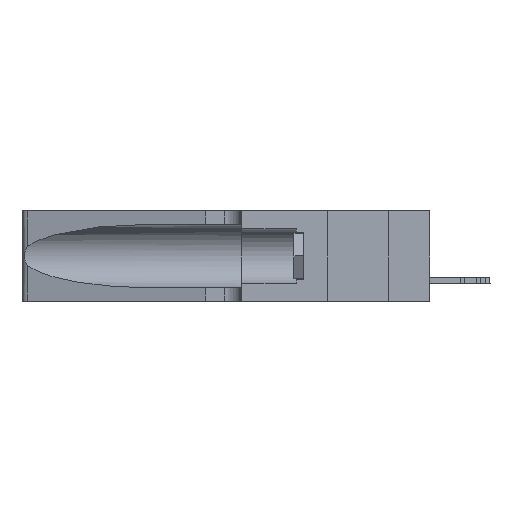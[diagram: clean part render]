
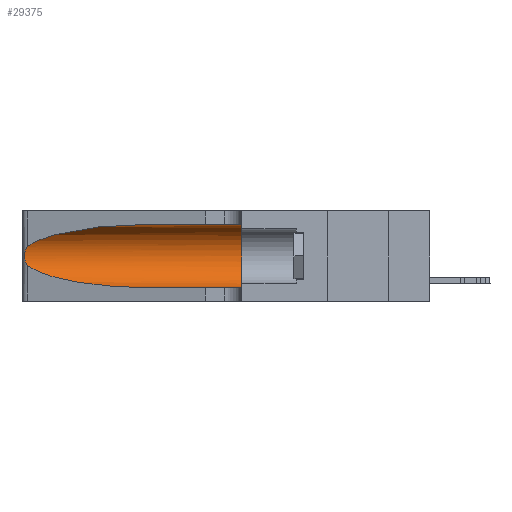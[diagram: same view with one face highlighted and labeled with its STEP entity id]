
A CAD part, left-side view. The second image highlights one B-rep face of the part: STEP entity #29375.
In plain terms, the highlighted cylindrical face has radius 3.308 mm (diameter 6.617 mm), a partial arc.
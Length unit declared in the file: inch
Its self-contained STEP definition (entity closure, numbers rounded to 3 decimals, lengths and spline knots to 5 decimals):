
#72 = CIRCLE ( 'NONE', #25936, 0.13025 ) ;
#590 =( BOUNDED_CURVE ( )  B_SPLINE_CURVE ( 3, ( #35340, #2138, #42446, #32160 ),
 .UNSPECIFIED., .F., .T. ) 
 B_SPLINE_CURVE_WITH_KNOTS ( ( 4, 4 ),
 ( 1.5708, 2.84003 ),
 .UNSPECIFIED. ) 
 CURVE ( )  GEOMETRIC_REPRESENTATION_ITEM ( )  RATIONAL_B_SPLINE_CURVE ( ( 1., 0.87, 0.87, 1. ) ) 
 REPRESENTATION_ITEM ( '' )  );
#1772 = CYLINDRICAL_SURFACE ( 'NONE', #24110, 0.13025 ) ;
#2138 = CARTESIAN_POINT ( 'NONE',  ( 0.18966, 0.96281, 0.31525 ) ) ;
#3364 = CARTESIAN_POINT ( 'NONE',  ( 0.26017, 1.23833, 0.17102 ) ) ;
#3553 = CARTESIAN_POINT ( 'NONE',  ( 0.1305, 0.72297, 0.05475 ) ) ;
#4095 = VERTEX_POINT ( 'NONE', #39929 ) ;
#5982 = CARTESIAN_POINT ( 'NONE',  ( 0.25639, 1.23184, 0.21858 ) ) ;
#6712 = CARTESIAN_POINT ( 'NONE',  ( 0.25787, 1.23484, 0.2124 ) ) ;
#8553 = B_SPLINE_CURVE_WITH_KNOTS ( 'NONE', 3,
 ( #29256, #28827, #5982, #6712, #12240, #23269, #42058, #12664, #3364, #29982, #9185, #25629, #38862, #39005 ),
 .UNSPECIFIED., .F., .F.,
 ( 4, 2, 2, 2, 2, 2, 4 ),
 ( 0., 0.00027, 0.00053, 0.00107, 0.0016, 0.00187, 0.00214 ),
 .UNSPECIFIED. ) ;
#9185 = CARTESIAN_POINT ( 'NONE',  ( 0.25789, 1.23486, 0.15765 ) ) ;
#10046 = CARTESIAN_POINT ( 'NONE',  ( 0.1305, 0.35, 0.05475 ) ) ;
#10356 = EDGE_CURVE ( 'NONE', #38696, #4095, #590, .T. ) ;
#10745 = CARTESIAN_POINT ( 'NONE',  ( 0.1305, 1.61858, 0.31525 ) ) ;
#10902 = CARTESIAN_POINT ( 'NONE',  ( 0.1305, 0.72297, 0.05475 ) ) ;
#11065 = VERTEX_POINT ( 'NONE', #10902 ) ;
#11170 = CARTESIAN_POINT ( 'NONE',  ( 0.1305, 1.61858, 0.05475 ) ) ;
#11509 = EDGE_CURVE ( 'NONE', #17687, #16863, #72, .T. ) ;
#11539 = DIRECTION ( 'NONE',  ( 0., 0., -1. ) ) ;
#12240 = CARTESIAN_POINT ( 'NONE',  ( 0.25854, 1.2359, 0.20912 ) ) ;
#12399 = ORIENTED_EDGE ( 'NONE', *, *, #41857, .T. ) ;
#12664 = CARTESIAN_POINT ( 'NONE',  ( 0.26075, 1.23896, 0.178 ) ) ;
#13166 = CARTESIAN_POINT ( 'NONE',  ( 0.25487, 1.22718, 0.14631 ) ) ;
#14409 = ORIENTED_EDGE ( 'NONE', *, *, #38711, .T. ) ;
#15258 = VERTEX_POINT ( 'NONE', #22957 ) ;
#16120 = CARTESIAN_POINT ( 'NONE',  ( 0.1305, 0.35, 0.31525 ) ) ;
#16863 = VERTEX_POINT ( 'NONE', #10046 ) ;
#17687 = VERTEX_POINT ( 'NONE', #16120 ) ;
#20116 = CARTESIAN_POINT ( 'NONE',  ( 0.18966, 0.96281, 0.05475 ) ) ;
#20128 = LINE ( 'NONE', #11170, #24814 ) ;
#21708 = CARTESIAN_POINT ( 'NONE',  ( 0.1305, 1.61858, 0.185 ) ) ;
#22957 = CARTESIAN_POINT ( 'NONE',  ( 0.25487, 1.22718, 0.14631 ) ) ;
#23132 = ORIENTED_EDGE ( 'NONE', *, *, #10356, .T. ) ;
#23269 = CARTESIAN_POINT ( 'NONE',  ( 0.26018, 1.23835, 0.19895 ) ) ;
#23907 = LINE ( 'NONE', #10745, #34899 ) ;
#24110 = AXIS2_PLACEMENT_3D ( 'NONE', #21708, #28264, #11539 ) ;
#24814 = VECTOR ( 'NONE', #37796, 39.37008 ) ;
#25629 = CARTESIAN_POINT ( 'NONE',  ( 0.25639, 1.23186, 0.15144 ) ) ;
#25936 = AXIS2_PLACEMENT_3D ( 'NONE', #38890, #28857, #35710 ) ;
#26674 = CARTESIAN_POINT ( 'NONE',  ( 0.2373, 1.15595, 0.08982 ) ) ;
#28264 = DIRECTION ( 'NONE',  ( 0., -1., 0. ) ) ;
#28827 = CARTESIAN_POINT ( 'NONE',  ( 0.25555, 1.22994, 0.2215 ) ) ;
#28857 = DIRECTION ( 'NONE',  ( 0., 1., 0. ) ) ;
#29256 = CARTESIAN_POINT ( 'NONE',  ( 0.25487, 1.22718, 0.22369 ) ) ;
#29375 = ADVANCED_FACE ( 'NONE', ( #35109 ), #1772, .F. ) ;
#29982 = CARTESIAN_POINT ( 'NONE',  ( 0.25856, 1.23593, 0.16098 ) ) ;
#31594 = CARTESIAN_POINT ( 'NONE',  ( 0.1305, 0.72297, 0.31525 ) ) ;
#32160 = CARTESIAN_POINT ( 'NONE',  ( 0.25487, 1.22718, 0.22369 ) ) ;
#34624 = EDGE_CURVE ( 'NONE', #38696, #17687, #23907, .T. ) ;
#34800 = ORIENTED_EDGE ( 'NONE', *, *, #40610, .T. ) ;
#34899 = VECTOR ( 'NONE', #41171, 39.37008 ) ;
#35109 = FACE_OUTER_BOUND ( 'NONE', #35824, .T. ) ;
#35340 = CARTESIAN_POINT ( 'NONE',  ( 0.1305, 0.72297, 0.31525 ) ) ;
#35710 = DIRECTION ( 'NONE',  ( 0., 0., 1. ) ) ;
#35798 =( BOUNDED_CURVE ( )  B_SPLINE_CURVE ( 3, ( #13166, #26674, #20116, #3553 ),
 .UNSPECIFIED., .F., .T. ) 
 B_SPLINE_CURVE_WITH_KNOTS ( ( 4, 4 ),
 ( 3.44316, 4.71239 ),
 .UNSPECIFIED. ) 
 CURVE ( )  GEOMETRIC_REPRESENTATION_ITEM ( )  RATIONAL_B_SPLINE_CURVE ( ( 1., 0.87, 0.87, 1. ) ) 
 REPRESENTATION_ITEM ( '' )  );
#35824 = EDGE_LOOP ( 'NONE', ( #23132, #34800, #12399, #14409, #39129, #36095 ) ) ;
#36095 = ORIENTED_EDGE ( 'NONE', *, *, #34624, .F. ) ;
#37796 = DIRECTION ( 'NONE',  ( 0., -1., 0. ) ) ;
#38696 = VERTEX_POINT ( 'NONE', #31594 ) ;
#38711 = EDGE_CURVE ( 'NONE', #11065, #16863, #20128, .T. ) ;
#38862 = CARTESIAN_POINT ( 'NONE',  ( 0.25555, 1.22993, 0.14849 ) ) ;
#38890 = CARTESIAN_POINT ( 'NONE',  ( 0.1305, 0.35, 0.185 ) ) ;
#39005 = CARTESIAN_POINT ( 'NONE',  ( 0.25487, 1.22718, 0.14631 ) ) ;
#39129 = ORIENTED_EDGE ( 'NONE', *, *, #11509, .F. ) ;
#39929 = CARTESIAN_POINT ( 'NONE',  ( 0.25487, 1.22718, 0.22369 ) ) ;
#40610 = EDGE_CURVE ( 'NONE', #4095, #15258, #8553, .T. ) ;
#41171 = DIRECTION ( 'NONE',  ( 0., -1., 0. ) ) ;
#41857 = EDGE_CURVE ( 'NONE', #15258, #11065, #35798, .T. ) ;
#42058 = CARTESIAN_POINT ( 'NONE',  ( 0.26075, 1.23896, 0.19203 ) ) ;
#42446 = CARTESIAN_POINT ( 'NONE',  ( 0.2373, 1.15595, 0.28018 ) ) ;
